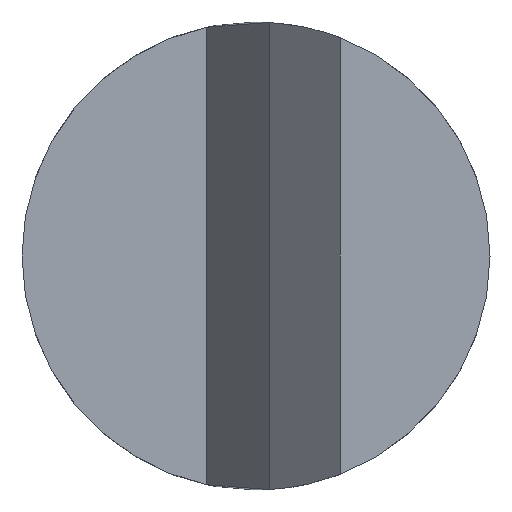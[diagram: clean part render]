
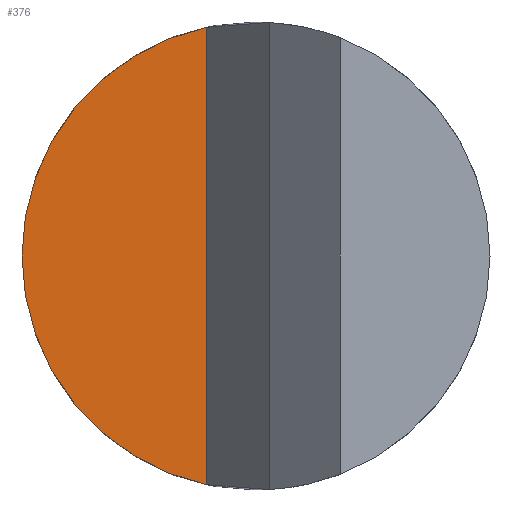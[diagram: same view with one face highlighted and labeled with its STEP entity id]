
A CAD part, left-side view. The second image highlights one B-rep face of the part: STEP entity #376.
In plain terms, the highlighted planar face has unit normal (-1, 0, 0).
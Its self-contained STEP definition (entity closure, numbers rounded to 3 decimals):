
#4 = VECTOR ( 'NONE', #31, 1000. ) ;
#19 = FACE_OUTER_BOUND ( 'NONE', #138, .T. ) ;
#21 = DIRECTION ( 'NONE',  ( 0., 1., 0. ) ) ;
#25 = VERTEX_POINT ( 'NONE', #123 ) ;
#29 = CARTESIAN_POINT ( 'NONE',  ( -6.49, 0.502, 0. ) ) ;
#31 = DIRECTION ( 'NONE',  ( 0., 0., 1. ) ) ;
#99 = LINE ( 'NONE', #29, #4 ) ;
#118 = DIRECTION ( 'NONE',  ( 1., 0., 0. ) ) ;
#121 = DIRECTION ( 'NONE',  ( 0., 1., 0. ) ) ;
#122 = DIRECTION ( 'NONE',  ( 1., 0., 0. ) ) ;
#123 = CARTESIAN_POINT ( 'NONE',  ( -6.49, 2.381, 0. ) ) ;
#127 = CARTESIAN_POINT ( 'NONE',  ( -6.49, 0., 0. ) ) ;
#138 = EDGE_LOOP ( 'NONE', ( #463, #307, #328 ) ) ;
#181 = DIRECTION ( 'NONE',  ( 0., 1., 0. ) ) ;
#184 = DIRECTION ( 'NONE',  ( 1., 0., 0. ) ) ;
#187 = CARTESIAN_POINT ( 'NONE',  ( -6.49, 0., 0. ) ) ;
#240 = AXIS2_PLACEMENT_3D ( 'NONE', #187, #184, #181 ) ;
#270 = AXIS2_PLACEMENT_3D ( 'NONE', #127, #122, #121 ) ;
#285 = CIRCLE ( 'NONE', #240, 2.381 ) ;
#307 = ORIENTED_EDGE ( 'NONE', *, *, #503, .T. ) ;
#328 = ORIENTED_EDGE ( 'NONE', *, *, #523, .F. ) ;
#330 = AXIS2_PLACEMENT_3D ( 'NONE', #399, #118, #21 ) ;
#351 = CIRCLE ( 'NONE', #270, 2.381 ) ;
#376 = ADVANCED_FACE ( 'NONE', ( #19 ), #403, .F. ) ;
#396 = VERTEX_POINT ( 'NONE', #587 ) ;
#399 = CARTESIAN_POINT ( 'NONE',  ( -6.49, 0.502, 0. ) ) ;
#403 = PLANE ( 'NONE',  #330 ) ;
#463 = ORIENTED_EDGE ( 'NONE', *, *, #491, .F. ) ;
#470 = VERTEX_POINT ( 'NONE', #532 ) ;
#491 = EDGE_CURVE ( 'NONE', #470, #25, #351, .T. ) ;
#503 = EDGE_CURVE ( 'NONE', #470, #396, #99, .T. ) ;
#523 = EDGE_CURVE ( 'NONE', #25, #396, #285, .T. ) ;
#532 = CARTESIAN_POINT ( 'NONE',  ( -6.49, 0.502, -2.328 ) ) ;
#587 = CARTESIAN_POINT ( 'NONE',  ( -6.49, 0.502, 2.328 ) ) ;
